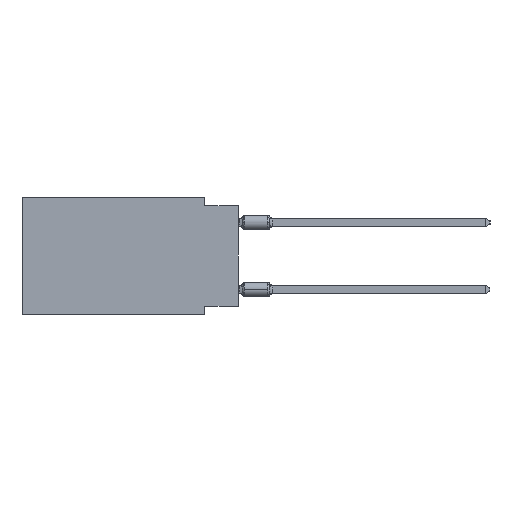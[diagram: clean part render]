
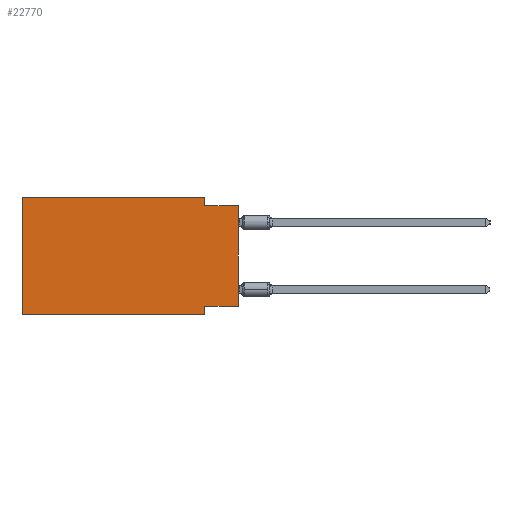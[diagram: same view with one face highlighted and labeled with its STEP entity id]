
A CAD part, left-side view. The second image highlights one B-rep face of the part: STEP entity #22770.
In plain terms, the highlighted planar face has unit normal (-1, 0, 0).
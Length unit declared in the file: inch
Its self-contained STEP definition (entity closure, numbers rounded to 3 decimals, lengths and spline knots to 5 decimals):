
#701 = ORIENTED_EDGE ( 'NONE', *, *, #21723, .T. ) ;
#857 = VECTOR ( 'NONE', #12041, 39.37008 ) ;
#1737 = LINE ( 'NONE', #28915, #3689 ) ;
#2597 = CARTESIAN_POINT ( 'NONE',  ( 0., 0.645, 0. ) ) ;
#2794 = CARTESIAN_POINT ( 'NONE',  ( 0., 0., -0.325 ) ) ;
#3172 = DIRECTION ( 'NONE',  ( 0., 1., 0. ) ) ;
#3577 = DIRECTION ( 'NONE',  ( 0., 0., -1. ) ) ;
#3623 = AXIS2_PLACEMENT_3D ( 'NONE', #20036, #29095, #4503 ) ;
#3689 = VECTOR ( 'NONE', #13779, 39.37008 ) ;
#4176 = LINE ( 'NONE', #33518, #30697 ) ;
#4503 = DIRECTION ( 'NONE',  ( 0., 0., -1. ) ) ;
#6510 = CARTESIAN_POINT ( 'NONE',  ( 0., 0.645, 0. ) ) ;
#6905 = CARTESIAN_POINT ( 'NONE',  ( 0., 0.645, 0. ) ) ;
#7514 = ORIENTED_EDGE ( 'NONE', *, *, #37758, .F. ) ;
#7827 = CARTESIAN_POINT ( 'NONE',  ( 0., 0.1, -0.025 ) ) ;
#8065 = CARTESIAN_POINT ( 'NONE',  ( 0., 0., -0.025 ) ) ;
#8809 = ORIENTED_EDGE ( 'NONE', *, *, #18060, .T. ) ;
#9467 = LINE ( 'NONE', #6510, #857 ) ;
#9557 = EDGE_CURVE ( 'NONE', #15389, #14358, #9467, .T. ) ;
#9754 = CARTESIAN_POINT ( 'NONE',  ( 0., 0., 0. ) ) ;
#9863 = EDGE_CURVE ( 'NONE', #31554, #34530, #31869, .T. ) ;
#10307 = CARTESIAN_POINT ( 'NONE',  ( 0., 0.645, -0.35 ) ) ;
#10563 = CARTESIAN_POINT ( 'NONE',  ( 0., 0., -0.325 ) ) ;
#12041 = DIRECTION ( 'NONE',  ( 0., -1., 0. ) ) ;
#12094 = VERTEX_POINT ( 'NONE', #10563 ) ;
#12872 = LINE ( 'NONE', #10307, #17997 ) ;
#13758 = ORIENTED_EDGE ( 'NONE', *, *, #9863, .F. ) ;
#13779 = DIRECTION ( 'NONE',  ( 0., 0., -1. ) ) ;
#13988 = ORIENTED_EDGE ( 'NONE', *, *, #28027, .F. ) ;
#14358 = VERTEX_POINT ( 'NONE', #17483 ) ;
#14544 = VECTOR ( 'NONE', #29557, 39.37008 ) ;
#14633 = LINE ( 'NONE', #2597, #14544 ) ;
#15389 = VERTEX_POINT ( 'NONE', #6905 ) ;
#16342 = FACE_OUTER_BOUND ( 'NONE', #37228, .T. ) ;
#17143 = VECTOR ( 'NONE', #3172, 39.37008 ) ;
#17483 = CARTESIAN_POINT ( 'NONE',  ( 0., 0.1, 0. ) ) ;
#17816 = CARTESIAN_POINT ( 'NONE',  ( 0., 0.1, -0.35 ) ) ;
#17847 = VECTOR ( 'NONE', #23378, 39.37008 ) ;
#17941 = VERTEX_POINT ( 'NONE', #17816 ) ;
#17997 = VECTOR ( 'NONE', #25631, 39.37008 ) ;
#18060 = EDGE_CURVE ( 'NONE', #12094, #34530, #34147, .T. ) ;
#20036 = CARTESIAN_POINT ( 'NONE',  ( 0., 0.645, 0. ) ) ;
#21723 = EDGE_CURVE ( 'NONE', #31884, #17941, #12872, .T. ) ;
#22770 = ADVANCED_FACE ( 'NONE', ( #16342 ), #34234, .F. ) ;
#23378 = DIRECTION ( 'NONE',  ( 0., -1., 0. ) ) ;
#23970 = EDGE_CURVE ( 'NONE', #37106, #17941, #1737, .T. ) ;
#24318 = ORIENTED_EDGE ( 'NONE', *, *, #30525, .F. ) ;
#25317 = CARTESIAN_POINT ( 'NONE',  ( 0., 0.1, -0.325 ) ) ;
#25631 = DIRECTION ( 'NONE',  ( 0., -1., 0. ) ) ;
#28027 = EDGE_CURVE ( 'NONE', #12094, #37106, #33092, .T. ) ;
#28915 = CARTESIAN_POINT ( 'NONE',  ( 0., 0.1, -0.35 ) ) ;
#28961 = ORIENTED_EDGE ( 'NONE', *, *, #23970, .F. ) ;
#29095 = DIRECTION ( 'NONE',  ( 1., 0., 0. ) ) ;
#29557 = DIRECTION ( 'NONE',  ( 0., 0., 1. ) ) ;
#30525 = EDGE_CURVE ( 'NONE', #14358, #31554, #4176, .T. ) ;
#30697 = VECTOR ( 'NONE', #3577, 39.37008 ) ;
#31182 = DIRECTION ( 'NONE',  ( 0., 0., 1. ) ) ;
#31403 = CARTESIAN_POINT ( 'NONE',  ( 0., 0.645, -0.35 ) ) ;
#31554 = VERTEX_POINT ( 'NONE', #7827 ) ;
#31642 = ORIENTED_EDGE ( 'NONE', *, *, #9557, .F. ) ;
#31869 = LINE ( 'NONE', #8065, #17847 ) ;
#31884 = VERTEX_POINT ( 'NONE', #31403 ) ;
#33092 = LINE ( 'NONE', #2794, #17143 ) ;
#33518 = CARTESIAN_POINT ( 'NONE',  ( 0., 0.1, 0. ) ) ;
#34147 = LINE ( 'NONE', #9754, #38187 ) ;
#34234 = PLANE ( 'NONE',  #3623 ) ;
#34530 = VERTEX_POINT ( 'NONE', #37693 ) ;
#37106 = VERTEX_POINT ( 'NONE', #25317 ) ;
#37228 = EDGE_LOOP ( 'NONE', ( #8809, #13758, #24318, #31642, #7514, #701, #28961, #13988 ) ) ;
#37693 = CARTESIAN_POINT ( 'NONE',  ( 0., 0., -0.025 ) ) ;
#37758 = EDGE_CURVE ( 'NONE', #31884, #15389, #14633, .T. ) ;
#38187 = VECTOR ( 'NONE', #31182, 39.37008 ) ;
